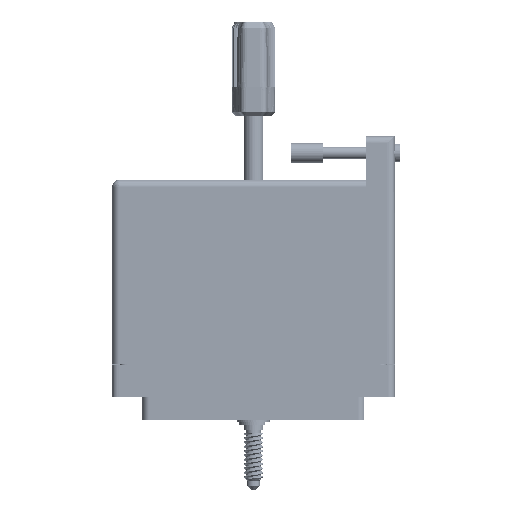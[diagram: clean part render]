
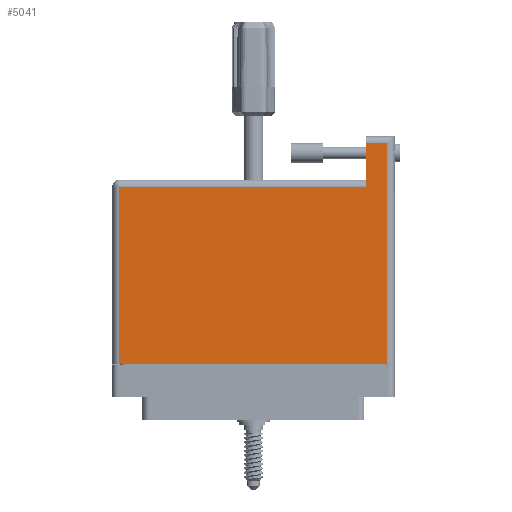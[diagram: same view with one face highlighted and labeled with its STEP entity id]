
A CAD part, front view. The second image highlights one B-rep face of the part: STEP entity #5041.
In plain terms, the highlighted face is planar.
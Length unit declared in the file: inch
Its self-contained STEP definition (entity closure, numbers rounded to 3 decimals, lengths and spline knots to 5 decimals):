
#952 = DIRECTION ( 'NONE',  ( 0., 0., -1. ) ) ;
#2450 = AXIS2_PLACEMENT_3D ( 'NONE', #80783, #952, #34064 ) ;
#2456 = CARTESIAN_POINT ( 'NONE',  ( 1.079, 2.095, 0.617 ) ) ;
#2979 = DIRECTION ( 'NONE',  ( 0., 1., 0. ) ) ;
#5041 = ADVANCED_FACE ( 'NONE', ( #81366 ), #20859, .F. ) ;
#8398 = LINE ( 'NONE', #41204, #53506 ) ;
#11177 = LINE ( 'NONE', #2456, #58407 ) ;
#12346 = CARTESIAN_POINT ( 'NONE',  ( -1.289, -0.1, 0.617 ) ) ;
#12634 = LINE ( 'NONE', #82772, #26328 ) ;
#14268 = VECTOR ( 'NONE', #31219, 39.37008 ) ;
#16078 = DIRECTION ( 'NONE',  ( 1., 0., 0. ) ) ;
#16859 = LINE ( 'NONE', #30534, #45284 ) ;
#20859 = PLANE ( 'NONE',  #2450 ) ;
#26328 = VECTOR ( 'NONE', #16078, 39.37008 ) ;
#26796 = DIRECTION ( 'NONE',  ( 0., -1., 0. ) ) ;
#27669 = EDGE_CURVE ( 'NONE', #58709, #71512, #12634, .T. ) ;
#29306 = EDGE_CURVE ( 'NONE', #75284, #60775, #8398, .T. ) ;
#30534 = CARTESIAN_POINT ( 'NONE',  ( 1.289, 2.095, 0.617 ) ) ;
#30775 = ORIENTED_EDGE ( 'NONE', *, *, #64857, .T. ) ;
#31219 = DIRECTION ( 'NONE',  ( -1., 0., 0. ) ) ;
#32085 = CARTESIAN_POINT ( 'NONE',  ( -1.359, 1.605, 0.617 ) ) ;
#33260 = EDGE_CURVE ( 'NONE', #60775, #73971, #11177, .T. ) ;
#34064 = DIRECTION ( 'NONE',  ( -1., 0., 0. ) ) ;
#34398 = CARTESIAN_POINT ( 'NONE',  ( -1.289, -0.1, 0.617 ) ) ;
#36048 = ORIENTED_EDGE ( 'NONE', *, *, #27669, .T. ) ;
#39453 = VERTEX_POINT ( 'NONE', #57506 ) ;
#41204 = CARTESIAN_POINT ( 'NONE',  ( -1.359, 2.025, 0.617 ) ) ;
#43637 = CARTESIAN_POINT ( 'NONE',  ( 1.079, 1.605, 0.617 ) ) ;
#45284 = VECTOR ( 'NONE', #2979, 39.37008 ) ;
#46906 = ORIENTED_EDGE ( 'NONE', *, *, #53566, .T. ) ;
#48602 = CARTESIAN_POINT ( 'NONE',  ( 1.079, 2.025, 0.617 ) ) ;
#53506 = VECTOR ( 'NONE', #54374, 39.37008 ) ;
#53566 = EDGE_CURVE ( 'NONE', #73971, #39453, #55243, .T. ) ;
#54374 = DIRECTION ( 'NONE',  ( -1., 0., 0. ) ) ;
#55194 = VECTOR ( 'NONE', #26796, 39.37008 ) ;
#55243 = LINE ( 'NONE', #32085, #14268 ) ;
#57506 = CARTESIAN_POINT ( 'NONE',  ( -1.289, 1.605, 0.617 ) ) ;
#58021 = EDGE_CURVE ( 'NONE', #71512, #75284, #16859, .T. ) ;
#58407 = VECTOR ( 'NONE', #62792, 39.37008 ) ;
#58709 = VERTEX_POINT ( 'NONE', #12346 ) ;
#60634 = ORIENTED_EDGE ( 'NONE', *, *, #58021, .T. ) ;
#60775 = VERTEX_POINT ( 'NONE', #48602 ) ;
#62792 = DIRECTION ( 'NONE',  ( 0., -1., 0. ) ) ;
#64753 = ORIENTED_EDGE ( 'NONE', *, *, #29306, .T. ) ;
#64857 = EDGE_CURVE ( 'NONE', #39453, #58709, #65559, .T. ) ;
#65559 = LINE ( 'NONE', #34398, #55194 ) ;
#67371 = EDGE_LOOP ( 'NONE', ( #46906, #30775, #36048, #60634, #64753, #80411 ) ) ;
#69370 = CARTESIAN_POINT ( 'NONE',  ( 1.289, 2.025, 0.617 ) ) ;
#71512 = VERTEX_POINT ( 'NONE', #75786 ) ;
#73971 = VERTEX_POINT ( 'NONE', #43637 ) ;
#75284 = VERTEX_POINT ( 'NONE', #69370 ) ;
#75786 = CARTESIAN_POINT ( 'NONE',  ( 1.289, -0.1, 0.617 ) ) ;
#80411 = ORIENTED_EDGE ( 'NONE', *, *, #33260, .T. ) ;
#80783 = CARTESIAN_POINT ( 'NONE',  ( -1.359, 1.675, 0.617 ) ) ;
#81366 = FACE_OUTER_BOUND ( 'NONE', #67371, .T. ) ;
#82772 = CARTESIAN_POINT ( 'NONE',  ( -1.359, -0.1, 0.617 ) ) ;
